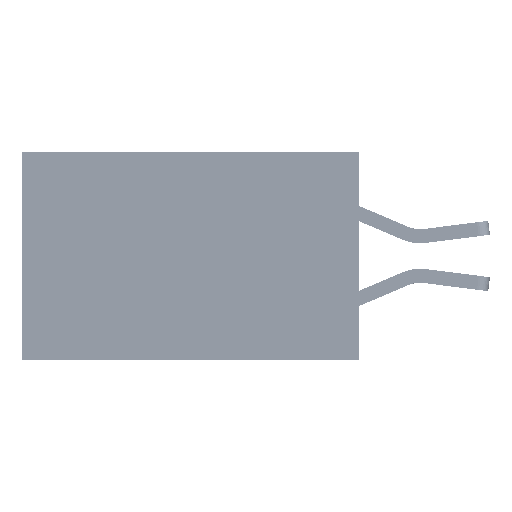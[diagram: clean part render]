
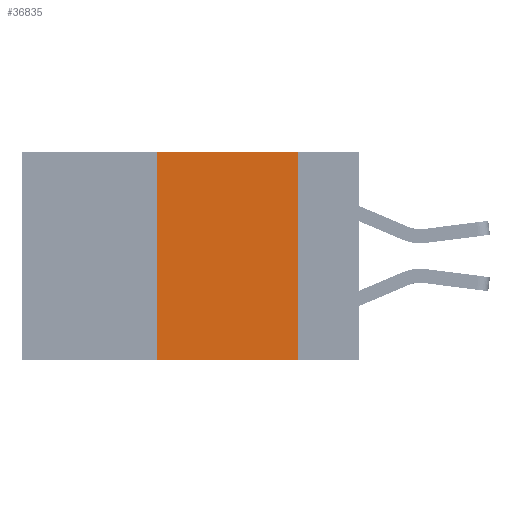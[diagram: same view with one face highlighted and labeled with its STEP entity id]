
A CAD part, left-side view. The second image highlights one B-rep face of the part: STEP entity #36835.
In plain terms, the highlighted planar face has unit normal (-1, 0, 0).
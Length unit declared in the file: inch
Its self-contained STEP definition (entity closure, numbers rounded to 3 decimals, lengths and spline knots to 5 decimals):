
#970 = VECTOR ( 'NONE', #5554, 39.37008 ) ;
#1728 = CARTESIAN_POINT ( 'NONE',  ( 0., 0.6, 0. ) ) ;
#4860 = CARTESIAN_POINT ( 'NONE',  ( 0., 0.36, -0.37 ) ) ;
#5554 = DIRECTION ( 'NONE',  ( 0., -1., 0. ) ) ;
#6296 = VERTEX_POINT ( 'NONE', #13000 ) ;
#7474 = EDGE_CURVE ( 'NONE', #6296, #17112, #8073, .T. ) ;
#8073 = LINE ( 'NONE', #1728, #970 ) ;
#9344 = ORIENTED_EDGE ( 'NONE', *, *, #19714, .T. ) ;
#12843 = PLANE ( 'NONE',  #22079 ) ;
#13000 = CARTESIAN_POINT ( 'NONE',  ( 0., 0.36, 0. ) ) ;
#13537 = ORIENTED_EDGE ( 'NONE', *, *, #7474, .F. ) ;
#14045 = CARTESIAN_POINT ( 'NONE',  ( 0., 0.11, -0.37 ) ) ;
#14792 = VERTEX_POINT ( 'NONE', #4860 ) ;
#17112 = VERTEX_POINT ( 'NONE', #17725 ) ;
#17160 = DIRECTION ( 'NONE',  ( 0., 0., 1. ) ) ;
#17725 = CARTESIAN_POINT ( 'NONE',  ( 0., 0.11, 0. ) ) ;
#17748 = LINE ( 'NONE', #23994, #18262 ) ;
#18262 = VECTOR ( 'NONE', #17160, 39.37008 ) ;
#18323 = EDGE_CURVE ( 'NONE', #17112, #28103, #21009, .T. ) ;
#19714 = EDGE_CURVE ( 'NONE', #14792, #28103, #37233, .T. ) ;
#20977 = DIRECTION ( 'NONE',  ( 0., 0., -1. ) ) ;
#21009 = LINE ( 'NONE', #41501, #23705 ) ;
#22079 = AXIS2_PLACEMENT_3D ( 'NONE', #41145, #40522, #30342 ) ;
#23705 = VECTOR ( 'NONE', #20977, 39.37008 ) ;
#23994 = CARTESIAN_POINT ( 'NONE',  ( 0., 0.36, 0. ) ) ;
#24090 = ORIENTED_EDGE ( 'NONE', *, *, #24932, .F. ) ;
#24862 = FACE_OUTER_BOUND ( 'NONE', #42621, .T. ) ;
#24932 = EDGE_CURVE ( 'NONE', #14792, #6296, #17748, .T. ) ;
#26086 = ORIENTED_EDGE ( 'NONE', *, *, #18323, .F. ) ;
#26669 = DIRECTION ( 'NONE',  ( 0., -1., 0. ) ) ;
#28103 = VERTEX_POINT ( 'NONE', #14045 ) ;
#30342 = DIRECTION ( 'NONE',  ( 0., 0., -1. ) ) ;
#33943 = VECTOR ( 'NONE', #26669, 39.37008 ) ;
#36835 = ADVANCED_FACE ( 'NONE', ( #24862 ), #12843, .F. ) ;
#37233 = LINE ( 'NONE', #44482, #33943 ) ;
#40522 = DIRECTION ( 'NONE',  ( 1., 0., 0. ) ) ;
#41145 = CARTESIAN_POINT ( 'NONE',  ( 0., 0.6, 0. ) ) ;
#41501 = CARTESIAN_POINT ( 'NONE',  ( 0., 0.11, 0. ) ) ;
#42621 = EDGE_LOOP ( 'NONE', ( #26086, #13537, #24090, #9344 ) ) ;
#44482 = CARTESIAN_POINT ( 'NONE',  ( 0., 0.6, -0.37 ) ) ;
